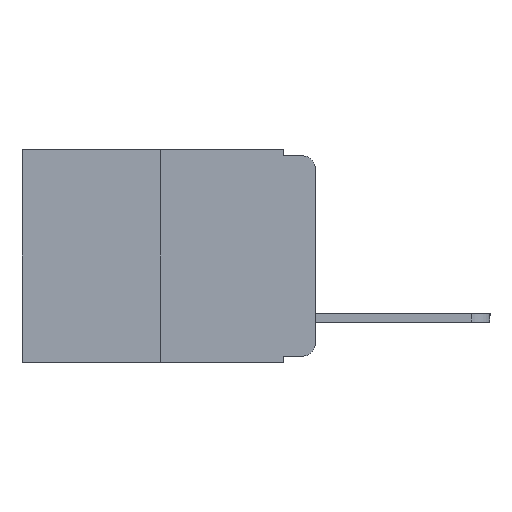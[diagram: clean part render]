
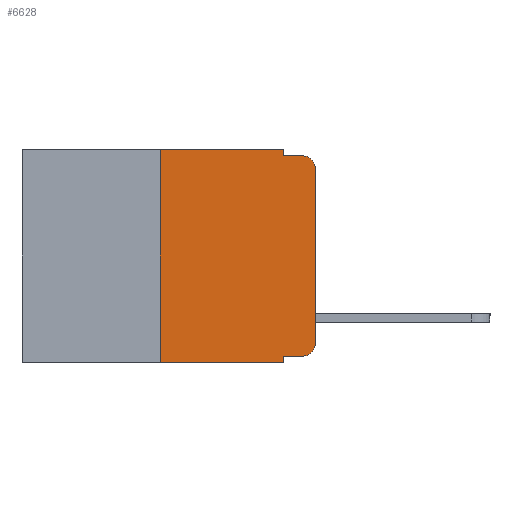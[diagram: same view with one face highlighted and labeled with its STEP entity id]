
A CAD part, left-side view. The second image highlights one B-rep face of the part: STEP entity #6628.
In plain terms, the highlighted planar face has unit normal (-1, 0, 0).
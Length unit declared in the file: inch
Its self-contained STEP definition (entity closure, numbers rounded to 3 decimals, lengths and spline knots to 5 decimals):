
#383 = VECTOR ( 'NONE', #10560, 39.37008 ) ;
#746 = EDGE_CURVE ( 'NONE', #10145, #6511, #23080, .T. ) ;
#878 = CARTESIAN_POINT ( 'NONE',  ( 0., 0.02, -0.333 ) ) ;
#971 = CARTESIAN_POINT ( 'NONE',  ( 0., 0.25, 0. ) ) ;
#1495 = DIRECTION ( 'NONE',  ( 0., 0., -1. ) ) ;
#1565 = DIRECTION ( 'NONE',  ( 0., 0., -1. ) ) ;
#1579 = VERTEX_POINT ( 'NONE', #11547 ) ;
#1764 = EDGE_CURVE ( 'NONE', #6640, #22307, #4448, .T. ) ;
#1785 = DIRECTION ( 'NONE',  ( 0., -1., 0. ) ) ;
#2035 = EDGE_CURVE ( 'NONE', #4168, #10145, #13629, .T. ) ;
#2400 = EDGE_LOOP ( 'NONE', ( #21846, #16501, #14988, #17287, #23870, #10672, #3549, #10226, #4832, #7408 ) ) ;
#2676 = VERTEX_POINT ( 'NONE', #11334 ) ;
#3169 = DIRECTION ( 'NONE',  ( -1., 0., 0. ) ) ;
#3340 = EDGE_CURVE ( 'NONE', #4168, #3644, #15527, .T. ) ;
#3539 = LINE ( 'NONE', #22132, #18049 ) ;
#3549 = ORIENTED_EDGE ( 'NONE', *, *, #20581, .T. ) ;
#3644 = VERTEX_POINT ( 'NONE', #3806 ) ;
#3806 = CARTESIAN_POINT ( 'NONE',  ( 0., 0.051, -0.343 ) ) ;
#4143 = VECTOR ( 'NONE', #18430, 39.37008 ) ;
#4168 = VERTEX_POINT ( 'NONE', #22264 ) ;
#4448 = LINE ( 'NONE', #19555, #13933 ) ;
#4615 = EDGE_CURVE ( 'NONE', #1579, #6640, #21651, .T. ) ;
#4832 = ORIENTED_EDGE ( 'NONE', *, *, #2035, .T. ) ;
#5258 = CARTESIAN_POINT ( 'NONE',  ( 0., 0.473, 0. ) ) ;
#5889 = EDGE_CURVE ( 'NONE', #22307, #2676, #17184, .T. ) ;
#5946 = FACE_OUTER_BOUND ( 'NONE', #2400, .T. ) ;
#6511 = VERTEX_POINT ( 'NONE', #10678 ) ;
#6628 = ADVANCED_FACE ( 'NONE', ( #5946 ), #20348, .F. ) ;
#6640 = VERTEX_POINT ( 'NONE', #7267 ) ;
#7179 = EDGE_CURVE ( 'NONE', #2676, #24120, #3539, .T. ) ;
#7267 = CARTESIAN_POINT ( 'NONE',  ( 0., 0.25, 0. ) ) ;
#7408 = ORIENTED_EDGE ( 'NONE', *, *, #746, .T. ) ;
#7575 = AXIS2_PLACEMENT_3D ( 'NONE', #24145, #12973, #1565 ) ;
#8476 = EDGE_CURVE ( 'NONE', #9264, #24120, #14137, .T. ) ;
#8886 = CARTESIAN_POINT ( 'NONE',  ( 0., 0.051, 0. ) ) ;
#9264 = VERTEX_POINT ( 'NONE', #13335 ) ;
#10145 = VERTEX_POINT ( 'NONE', #878 ) ;
#10226 = ORIENTED_EDGE ( 'NONE', *, *, #3340, .F. ) ;
#10560 = DIRECTION ( 'NONE',  ( 0., 0., -1. ) ) ;
#10672 = ORIENTED_EDGE ( 'NONE', *, *, #4615, .F. ) ;
#10678 = CARTESIAN_POINT ( 'NONE',  ( 0., 0., -0.313 ) ) ;
#10781 = CARTESIAN_POINT ( 'NONE',  ( 0., 0.051, -0.333 ) ) ;
#11011 = EDGE_CURVE ( 'NONE', #6511, #9264, #16735, .T. ) ;
#11140 = DIRECTION ( 'NONE',  ( 0., 0., 1. ) ) ;
#11334 = CARTESIAN_POINT ( 'NONE',  ( 0., 0.051, -0.01 ) ) ;
#11547 = CARTESIAN_POINT ( 'NONE',  ( 0., 0.25, -0.343 ) ) ;
#12267 = VECTOR ( 'NONE', #12407, 39.37008 ) ;
#12342 = VECTOR ( 'NONE', #11140, 39.37008 ) ;
#12407 = DIRECTION ( 'NONE',  ( 0., 0., 1. ) ) ;
#12906 = DIRECTION ( 'NONE',  ( 1., 0., 0. ) ) ;
#12973 = DIRECTION ( 'NONE',  ( -1., 0., 0. ) ) ;
#13335 = CARTESIAN_POINT ( 'NONE',  ( 0., 0., -0.03 ) ) ;
#13533 = AXIS2_PLACEMENT_3D ( 'NONE', #14520, #3169, #16416 ) ;
#13629 = LINE ( 'NONE', #10781, #4143 ) ;
#13933 = VECTOR ( 'NONE', #23313, 39.37008 ) ;
#14137 = CIRCLE ( 'NONE', #13533, 0.02 ) ;
#14198 = VECTOR ( 'NONE', #1785, 39.37008 ) ;
#14520 = CARTESIAN_POINT ( 'NONE',  ( 0., 0.02, -0.03 ) ) ;
#14988 = ORIENTED_EDGE ( 'NONE', *, *, #7179, .F. ) ;
#15527 = LINE ( 'NONE', #21805, #383 ) ;
#16231 = CARTESIAN_POINT ( 'NONE',  ( 0., 0.02, -0.01 ) ) ;
#16240 = CARTESIAN_POINT ( 'NONE',  ( 0., 0.051, 0. ) ) ;
#16330 = AXIS2_PLACEMENT_3D ( 'NONE', #5258, #12906, #1495 ) ;
#16416 = DIRECTION ( 'NONE',  ( 0., 0., -1. ) ) ;
#16501 = ORIENTED_EDGE ( 'NONE', *, *, #8476, .T. ) ;
#16735 = LINE ( 'NONE', #24192, #12342 ) ;
#17184 = LINE ( 'NONE', #8886, #23322 ) ;
#17287 = ORIENTED_EDGE ( 'NONE', *, *, #5889, .F. ) ;
#18049 = VECTOR ( 'NONE', #23976, 39.37008 ) ;
#18430 = DIRECTION ( 'NONE',  ( 0., -1., 0. ) ) ;
#19555 = CARTESIAN_POINT ( 'NONE',  ( 0., 0.473, 0. ) ) ;
#19773 = LINE ( 'NONE', #22533, #14198 ) ;
#20138 = DIRECTION ( 'NONE',  ( 0., 0., -1. ) ) ;
#20348 = PLANE ( 'NONE',  #16330 ) ;
#20581 = EDGE_CURVE ( 'NONE', #1579, #3644, #19773, .T. ) ;
#21651 = LINE ( 'NONE', #971, #12267 ) ;
#21805 = CARTESIAN_POINT ( 'NONE',  ( 0., 0.051, 0. ) ) ;
#21846 = ORIENTED_EDGE ( 'NONE', *, *, #11011, .T. ) ;
#22132 = CARTESIAN_POINT ( 'NONE',  ( 0., 0.051, -0.01 ) ) ;
#22264 = CARTESIAN_POINT ( 'NONE',  ( 0., 0.051, -0.333 ) ) ;
#22307 = VERTEX_POINT ( 'NONE', #16240 ) ;
#22533 = CARTESIAN_POINT ( 'NONE',  ( 0., 0.473, -0.343 ) ) ;
#23080 = CIRCLE ( 'NONE', #7575, 0.02 ) ;
#23313 = DIRECTION ( 'NONE',  ( 0., -1., 0. ) ) ;
#23322 = VECTOR ( 'NONE', #20138, 39.37008 ) ;
#23870 = ORIENTED_EDGE ( 'NONE', *, *, #1764, .F. ) ;
#23976 = DIRECTION ( 'NONE',  ( 0., -1., 0. ) ) ;
#24120 = VERTEX_POINT ( 'NONE', #16231 ) ;
#24145 = CARTESIAN_POINT ( 'NONE',  ( 0., 0.02, -0.313 ) ) ;
#24192 = CARTESIAN_POINT ( 'NONE',  ( 0., 0., 0. ) ) ;
